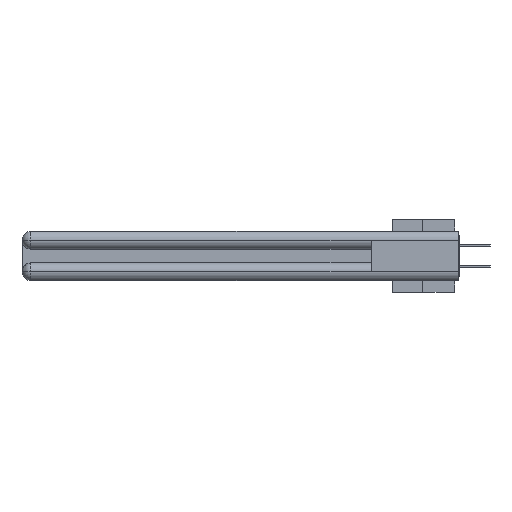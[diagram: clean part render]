
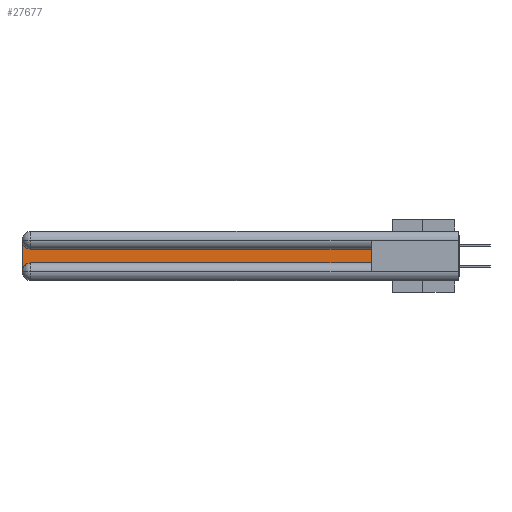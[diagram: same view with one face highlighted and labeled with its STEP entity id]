
A CAD part, left-side view. The second image highlights one B-rep face of the part: STEP entity #27677.
In plain terms, the highlighted planar face has unit normal (-1, 0, 0).
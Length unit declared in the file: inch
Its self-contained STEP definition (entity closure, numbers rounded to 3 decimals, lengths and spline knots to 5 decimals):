
#113 = CARTESIAN_POINT ( 'NONE',  ( 0.075, 2.94, -0.1225 ) ) ;
#115 = EDGE_CURVE ( 'NONE', #12537, #32377, #35123, .T. ) ;
#138 = EDGE_CURVE ( 'NONE', #605, #12537, #12725, .T. ) ;
#151 = CARTESIAN_POINT ( 'NONE',  ( 0.075, 2.94, -0.2175 ) ) ;
#605 = VERTEX_POINT ( 'NONE', #113 ) ;
#1338 = CARTESIAN_POINT ( 'NONE',  ( 0.075, 2.94, -0.2775 ) ) ;
#1573 = ORIENTED_EDGE ( 'NONE', *, *, #28075, .T. ) ;
#2045 = CARTESIAN_POINT ( 'NONE',  ( 0.075, 3., -0.0625 ) ) ;
#3577 = PLANE ( 'NONE',  #25591 ) ;
#4221 = LINE ( 'NONE', #8743, #15658 ) ;
#5173 = VECTOR ( 'NONE', #33539, 39.37008 ) ;
#5975 = EDGE_CURVE ( 'NONE', #26456, #20582, #4221, .T. ) ;
#6063 = DIRECTION ( 'NONE',  ( 0., 0., -1. ) ) ;
#8612 = DIRECTION ( 'NONE',  ( 0., 0., 1. ) ) ;
#8743 = CARTESIAN_POINT ( 'NONE',  ( 0.075, 0.6, -0.2175 ) ) ;
#11048 = ORIENTED_EDGE ( 'NONE', *, *, #115, .T. ) ;
#11376 = DIRECTION ( 'NONE',  ( 0., 1., 0. ) ) ;
#12185 = AXIS2_PLACEMENT_3D ( 'NONE', #14621, #19881, #23070 ) ;
#12537 = VERTEX_POINT ( 'NONE', #2045 ) ;
#12725 = CIRCLE ( 'NONE', #12185, 0.06 ) ;
#13579 = VERTEX_POINT ( 'NONE', #151 ) ;
#13884 = CARTESIAN_POINT ( 'NONE',  ( 0.075, 0.6, -0.2175 ) ) ;
#14243 = DIRECTION ( 'NONE',  ( 0., 0., -1. ) ) ;
#14621 = CARTESIAN_POINT ( 'NONE',  ( 0.075, 2.94, -0.0625 ) ) ;
#14653 = EDGE_CURVE ( 'NONE', #32377, #13579, #23536, .T. ) ;
#14907 = VECTOR ( 'NONE', #14243, 39.37008 ) ;
#15606 = DIRECTION ( 'NONE',  ( 0., 0., -1. ) ) ;
#15658 = VECTOR ( 'NONE', #8612, 39.37008 ) ;
#18894 = ORIENTED_EDGE ( 'NONE', *, *, #138, .T. ) ;
#19881 = DIRECTION ( 'NONE',  ( 1., 0., 0. ) ) ;
#20582 = VERTEX_POINT ( 'NONE', #29541 ) ;
#21153 = DIRECTION ( 'NONE',  ( 1., 0., 0. ) ) ;
#22329 = FACE_OUTER_BOUND ( 'NONE', #29952, .T. ) ;
#22855 = CARTESIAN_POINT ( 'NONE',  ( 0.075, 3., -0.1225 ) ) ;
#23070 = DIRECTION ( 'NONE',  ( 0., 0., -1. ) ) ;
#23536 = CIRCLE ( 'NONE', #26937, 0.06 ) ;
#24913 = CARTESIAN_POINT ( 'NONE',  ( 0.075, 0.6, -0.2175 ) ) ;
#25320 = LINE ( 'NONE', #31484, #30119 ) ;
#25591 = AXIS2_PLACEMENT_3D ( 'NONE', #22855, #28258, #6063 ) ;
#26456 = VERTEX_POINT ( 'NONE', #24913 ) ;
#26748 = CARTESIAN_POINT ( 'NONE',  ( 0.075, 3., -0.2775 ) ) ;
#26937 = AXIS2_PLACEMENT_3D ( 'NONE', #1338, #21153, #15606 ) ;
#27075 = ORIENTED_EDGE ( 'NONE', *, *, #5975, .T. ) ;
#27677 = ADVANCED_FACE ( 'NONE', ( #22329 ), #3577, .F. ) ;
#28075 = EDGE_CURVE ( 'NONE', #13579, #26456, #36357, .T. ) ;
#28258 = DIRECTION ( 'NONE',  ( 1., 0., 0. ) ) ;
#29052 = EDGE_CURVE ( 'NONE', #20582, #605, #25320, .T. ) ;
#29541 = CARTESIAN_POINT ( 'NONE',  ( 0.075, 0.6, -0.1225 ) ) ;
#29952 = EDGE_LOOP ( 'NONE', ( #35838, #18894, #11048, #33896, #1573, #27075 ) ) ;
#30119 = VECTOR ( 'NONE', #11376, 39.37008 ) ;
#31484 = CARTESIAN_POINT ( 'NONE',  ( 0.075, 0.6, -0.1225 ) ) ;
#32377 = VERTEX_POINT ( 'NONE', #26748 ) ;
#33539 = DIRECTION ( 'NONE',  ( 0., -1., 0. ) ) ;
#33896 = ORIENTED_EDGE ( 'NONE', *, *, #14653, .T. ) ;
#34291 = CARTESIAN_POINT ( 'NONE',  ( 0.075, 3., -0.2175 ) ) ;
#35123 = LINE ( 'NONE', #34291, #14907 ) ;
#35838 = ORIENTED_EDGE ( 'NONE', *, *, #29052, .T. ) ;
#36357 = LINE ( 'NONE', #13884, #5173 ) ;
